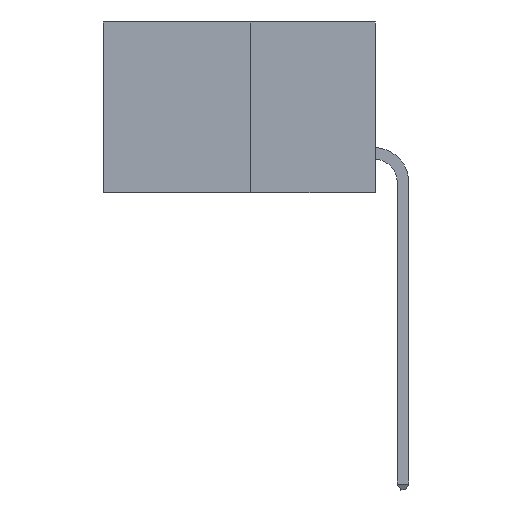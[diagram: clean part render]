
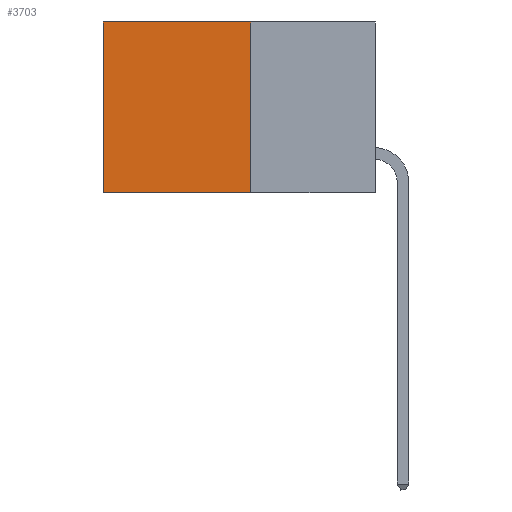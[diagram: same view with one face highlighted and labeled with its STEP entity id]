
A CAD part, left-side view. The second image highlights one B-rep face of the part: STEP entity #3703.
In plain terms, the highlighted planar face has unit normal (-1, 0, 0).
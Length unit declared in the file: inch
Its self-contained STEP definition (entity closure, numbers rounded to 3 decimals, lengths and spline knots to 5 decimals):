
#77 = VERTEX_POINT ( 'NONE', #7802 ) ;
#342 = CARTESIAN_POINT ( 'NONE',  ( 0.277, 0.27, -0.37 ) ) ;
#495 = ORIENTED_EDGE ( 'NONE', *, *, #2331, .T. ) ;
#1068 = DIRECTION ( 'NONE',  ( 0., 1., 0. ) ) ;
#1662 = CARTESIAN_POINT ( 'NONE',  ( 0.277, 0.59, 0. ) ) ;
#2219 = FACE_OUTER_BOUND ( 'NONE', #8272, .T. ) ;
#2331 = EDGE_CURVE ( 'NONE', #5278, #9000, #5843, .T. ) ;
#2510 = VECTOR ( 'NONE', #7692, 39.37008 ) ;
#3021 = CARTESIAN_POINT ( 'NONE',  ( 0.277, 0.59, -0.37 ) ) ;
#3129 = CARTESIAN_POINT ( 'NONE',  ( 0.277, 0.27, -0.37 ) ) ;
#3703 = ADVANCED_FACE ( 'NONE', ( #2219 ), #11982, .F. ) ;
#4055 = DIRECTION ( 'NONE',  ( 0., 0., -1. ) ) ;
#4723 = DIRECTION ( 'NONE',  ( 0., 0., -1. ) ) ;
#4838 = VERTEX_POINT ( 'NONE', #5147 ) ;
#5147 = CARTESIAN_POINT ( 'NONE',  ( 0.277, 0.59, -0.37 ) ) ;
#5163 = VECTOR ( 'NONE', #4723, 39.37008 ) ;
#5278 = VERTEX_POINT ( 'NONE', #9385 ) ;
#5843 = LINE ( 'NONE', #11874, #2510 ) ;
#6760 = LINE ( 'NONE', #3021, #11689 ) ;
#6847 = EDGE_CURVE ( 'NONE', #5278, #77, #12381, .T. ) ;
#7075 = ORIENTED_EDGE ( 'NONE', *, *, #9599, .T. ) ;
#7692 = DIRECTION ( 'NONE',  ( 0., 1., 0. ) ) ;
#7802 = CARTESIAN_POINT ( 'NONE',  ( 0.277, 0.27, -0.37 ) ) ;
#8272 = EDGE_LOOP ( 'NONE', ( #7075, #10773, #9658, #495 ) ) ;
#8983 = DIRECTION ( 'NONE',  ( 1., 0., 0. ) ) ;
#9000 = VERTEX_POINT ( 'NONE', #1662 ) ;
#9253 = DIRECTION ( 'NONE',  ( 0., 0., -1. ) ) ;
#9294 = VECTOR ( 'NONE', #1068, 39.37008 ) ;
#9385 = CARTESIAN_POINT ( 'NONE',  ( 0.277, 0.27, 0. ) ) ;
#9599 = EDGE_CURVE ( 'NONE', #9000, #4838, #6760, .T. ) ;
#9658 = ORIENTED_EDGE ( 'NONE', *, *, #6847, .F. ) ;
#9840 = AXIS2_PLACEMENT_3D ( 'NONE', #342, #8983, #9253 ) ;
#10772 = CARTESIAN_POINT ( 'NONE',  ( 0.277, 0.27, -0.37 ) ) ;
#10773 = ORIENTED_EDGE ( 'NONE', *, *, #10885, .F. ) ;
#10885 = EDGE_CURVE ( 'NONE', #77, #4838, #11657, .T. ) ;
#11657 = LINE ( 'NONE', #3129, #9294 ) ;
#11689 = VECTOR ( 'NONE', #4055, 39.37008 ) ;
#11874 = CARTESIAN_POINT ( 'NONE',  ( 0.277, 0.27, 0. ) ) ;
#11982 = PLANE ( 'NONE',  #9840 ) ;
#12381 = LINE ( 'NONE', #10772, #5163 ) ;
